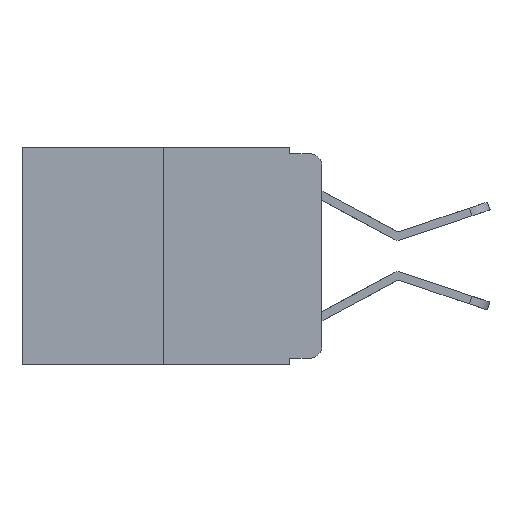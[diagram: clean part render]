
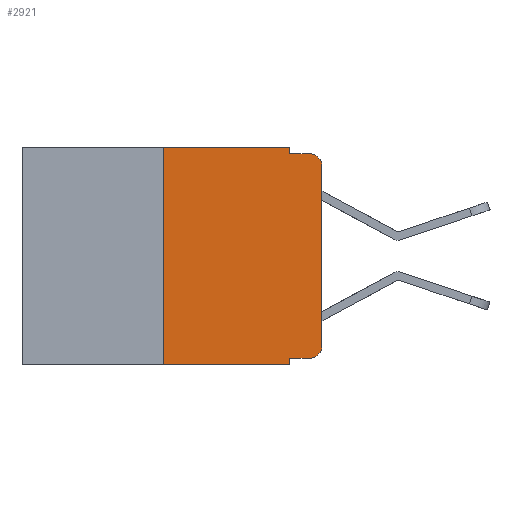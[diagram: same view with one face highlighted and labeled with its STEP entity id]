
A CAD part, left-side view. The second image highlights one B-rep face of the part: STEP entity #2921.
In plain terms, the highlighted planar face has unit normal (-1, 0, 0).
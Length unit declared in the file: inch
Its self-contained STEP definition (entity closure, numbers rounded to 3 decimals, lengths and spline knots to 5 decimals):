
#60 = ORIENTED_EDGE ( 'NONE', *, *, #13312, .T. ) ;
#237 = LINE ( 'NONE', #6367, #5695 ) ;
#402 = CARTESIAN_POINT ( 'NONE',  ( 0., 0., -0.313 ) ) ;
#577 = DIRECTION ( 'NONE',  ( 0., 0., -1. ) ) ;
#618 = CARTESIAN_POINT ( 'NONE',  ( 0., 0.051, -0.333 ) ) ;
#791 = LINE ( 'NONE', #2284, #3358 ) ;
#805 = ORIENTED_EDGE ( 'NONE', *, *, #910, .F. ) ;
#910 = EDGE_CURVE ( 'NONE', #13393, #6838, #5749, .T. ) ;
#1187 = CARTESIAN_POINT ( 'NONE',  ( 0., 0.25, -0.343 ) ) ;
#1193 = DIRECTION ( 'NONE',  ( 0., 0., 1. ) ) ;
#1488 = VERTEX_POINT ( 'NONE', #6975 ) ;
#1677 = ORIENTED_EDGE ( 'NONE', *, *, #7303, .T. ) ;
#1845 = DIRECTION ( 'NONE',  ( -1., 0., 0. ) ) ;
#1857 = VECTOR ( 'NONE', #5152, 39.37008 ) ;
#2062 = DIRECTION ( 'NONE',  ( 0., -1., 0. ) ) ;
#2085 = LINE ( 'NONE', #5122, #4639 ) ;
#2284 = CARTESIAN_POINT ( 'NONE',  ( 0., 0., 0. ) ) ;
#2587 = VERTEX_POINT ( 'NONE', #3376 ) ;
#2588 = VERTEX_POINT ( 'NONE', #1187 ) ;
#2653 = AXIS2_PLACEMENT_3D ( 'NONE', #8204, #1845, #9225 ) ;
#2921 = ADVANCED_FACE ( 'NONE', ( #11603 ), #11415, .F. ) ;
#3061 = DIRECTION ( 'NONE',  ( 0., -1., 0. ) ) ;
#3358 = VECTOR ( 'NONE', #1193, 39.37008 ) ;
#3376 = CARTESIAN_POINT ( 'NONE',  ( 0., 0.02, -0.01 ) ) ;
#3905 = VECTOR ( 'NONE', #4027, 39.37008 ) ;
#3956 = CARTESIAN_POINT ( 'NONE',  ( 0., 0.473, 0. ) ) ;
#4027 = DIRECTION ( 'NONE',  ( 0., 0., -1. ) ) ;
#4045 = ORIENTED_EDGE ( 'NONE', *, *, #7485, .T. ) ;
#4062 = CARTESIAN_POINT ( 'NONE',  ( 0., 0.051, -0.01 ) ) ;
#4426 = AXIS2_PLACEMENT_3D ( 'NONE', #7372, #12424, #6376 ) ;
#4442 = CARTESIAN_POINT ( 'NONE',  ( 0., 0.051, -0.343 ) ) ;
#4639 = VECTOR ( 'NONE', #6215, 39.37008 ) ;
#4798 = VECTOR ( 'NONE', #9281, 39.37008 ) ;
#5121 = LINE ( 'NONE', #11240, #4798 ) ;
#5122 = CARTESIAN_POINT ( 'NONE',  ( 0., 0.051, 0. ) ) ;
#5152 = DIRECTION ( 'NONE',  ( 0., -1., 0. ) ) ;
#5291 = VERTEX_POINT ( 'NONE', #7695 ) ;
#5512 = CARTESIAN_POINT ( 'NONE',  ( 0., 0.051, 0. ) ) ;
#5682 = VECTOR ( 'NONE', #13073, 39.37008 ) ;
#5695 = VECTOR ( 'NONE', #2062, 39.37008 ) ;
#5749 = LINE ( 'NONE', #3956, #12869 ) ;
#6215 = DIRECTION ( 'NONE',  ( 0., 0., -1. ) ) ;
#6367 = CARTESIAN_POINT ( 'NONE',  ( 0., 0.473, -0.343 ) ) ;
#6376 = DIRECTION ( 'NONE',  ( 0., 0., -1. ) ) ;
#6635 = CARTESIAN_POINT ( 'NONE',  ( 0., 0.051, -0.333 ) ) ;
#6838 = VERTEX_POINT ( 'NONE', #5512 ) ;
#6975 = CARTESIAN_POINT ( 'NONE',  ( 0., 0.051, -0.01 ) ) ;
#7055 = DIRECTION ( 'NONE',  ( -1., 0., 0. ) ) ;
#7303 = EDGE_CURVE ( 'NONE', #7454, #9127, #13252, .T. ) ;
#7372 = CARTESIAN_POINT ( 'NONE',  ( 0., 0.473, 0. ) ) ;
#7454 = VERTEX_POINT ( 'NONE', #13323 ) ;
#7483 = EDGE_LOOP ( 'NONE', ( #60, #8621, #13423, #9413, #805, #8332, #4045, #10549, #13284, #1677 ) ) ;
#7485 = EDGE_CURVE ( 'NONE', #2588, #8974, #237, .T. ) ;
#7559 = LINE ( 'NONE', #4062, #1857 ) ;
#7695 = CARTESIAN_POINT ( 'NONE',  ( 0., 0., -0.03 ) ) ;
#7996 = EDGE_CURVE ( 'NONE', #10292, #7454, #11410, .T. ) ;
#8204 = CARTESIAN_POINT ( 'NONE',  ( 0., 0.02, -0.313 ) ) ;
#8223 = CARTESIAN_POINT ( 'NONE',  ( 0., 0.051, 0. ) ) ;
#8332 = ORIENTED_EDGE ( 'NONE', *, *, #9341, .F. ) ;
#8621 = ORIENTED_EDGE ( 'NONE', *, *, #12027, .T. ) ;
#8683 = EDGE_CURVE ( 'NONE', #10292, #8974, #2085, .T. ) ;
#8974 = VERTEX_POINT ( 'NONE', #4442 ) ;
#9127 = VERTEX_POINT ( 'NONE', #402 ) ;
#9225 = DIRECTION ( 'NONE',  ( 0., 0., -1. ) ) ;
#9281 = DIRECTION ( 'NONE',  ( 0., 0., 1. ) ) ;
#9341 = EDGE_CURVE ( 'NONE', #2588, #13393, #5121, .T. ) ;
#9413 = ORIENTED_EDGE ( 'NONE', *, *, #10701, .F. ) ;
#10292 = VERTEX_POINT ( 'NONE', #6635 ) ;
#10546 = AXIS2_PLACEMENT_3D ( 'NONE', #13043, #7055, #577 ) ;
#10549 = ORIENTED_EDGE ( 'NONE', *, *, #8683, .F. ) ;
#10701 = EDGE_CURVE ( 'NONE', #6838, #1488, #12123, .T. ) ;
#11240 = CARTESIAN_POINT ( 'NONE',  ( 0., 0.25, 0. ) ) ;
#11359 = EDGE_CURVE ( 'NONE', #1488, #2587, #7559, .T. ) ;
#11410 = LINE ( 'NONE', #618, #5682 ) ;
#11415 = PLANE ( 'NONE',  #4426 ) ;
#11489 = CIRCLE ( 'NONE', #10546, 0.02 ) ;
#11603 = FACE_OUTER_BOUND ( 'NONE', #7483, .T. ) ;
#12027 = EDGE_CURVE ( 'NONE', #5291, #2587, #11489, .T. ) ;
#12123 = LINE ( 'NONE', #8223, #3905 ) ;
#12424 = DIRECTION ( 'NONE',  ( 1., 0., 0. ) ) ;
#12738 = CARTESIAN_POINT ( 'NONE',  ( 0., 0.25, 0. ) ) ;
#12869 = VECTOR ( 'NONE', #3061, 39.37008 ) ;
#13043 = CARTESIAN_POINT ( 'NONE',  ( 0., 0.02, -0.03 ) ) ;
#13073 = DIRECTION ( 'NONE',  ( 0., -1., 0. ) ) ;
#13252 = CIRCLE ( 'NONE', #2653, 0.02 ) ;
#13284 = ORIENTED_EDGE ( 'NONE', *, *, #7996, .T. ) ;
#13312 = EDGE_CURVE ( 'NONE', #9127, #5291, #791, .T. ) ;
#13323 = CARTESIAN_POINT ( 'NONE',  ( 0., 0.02, -0.333 ) ) ;
#13393 = VERTEX_POINT ( 'NONE', #12738 ) ;
#13423 = ORIENTED_EDGE ( 'NONE', *, *, #11359, .F. ) ;
